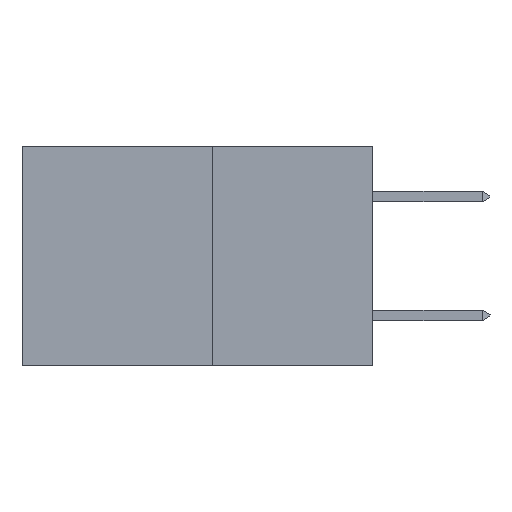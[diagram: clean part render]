
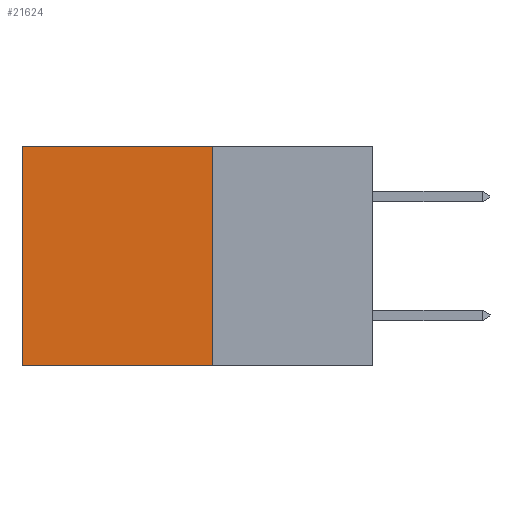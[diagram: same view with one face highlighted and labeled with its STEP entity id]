
A CAD part, left-side view. The second image highlights one B-rep face of the part: STEP entity #21624.
In plain terms, the highlighted planar face has unit normal (-1, 0, 0).
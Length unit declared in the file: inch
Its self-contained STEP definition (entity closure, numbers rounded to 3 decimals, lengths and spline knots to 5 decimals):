
#199 = CARTESIAN_POINT ( 'NONE',  ( 0.277, 0.27, 0. ) ) ;
#766 = EDGE_CURVE ( 'NONE', #6786, #12776, #12667, .T. ) ;
#1552 = DIRECTION ( 'NONE',  ( 0., 1., 0. ) ) ;
#2279 = VECTOR ( 'NONE', #3803, 39.37008 ) ;
#3022 = CARTESIAN_POINT ( 'NONE',  ( 0.277, 0.27, -0.37 ) ) ;
#3259 = CARTESIAN_POINT ( 'NONE',  ( 0.277, 0.27, 0. ) ) ;
#3731 = VECTOR ( 'NONE', #17454, 39.37008 ) ;
#3803 = DIRECTION ( 'NONE',  ( 0., 1., 0. ) ) ;
#4736 = PLANE ( 'NONE',  #23978 ) ;
#4869 = CARTESIAN_POINT ( 'NONE',  ( 0.277, 0.59, -0.37 ) ) ;
#4876 = CARTESIAN_POINT ( 'NONE',  ( 0.277, 0.27, -0.37 ) ) ;
#5575 = ORIENTED_EDGE ( 'NONE', *, *, #766, .T. ) ;
#6635 = DIRECTION ( 'NONE',  ( 0., 0., -1. ) ) ;
#6786 = VERTEX_POINT ( 'NONE', #3259 ) ;
#6839 = EDGE_CURVE ( 'NONE', #16352, #12604, #13921, .T. ) ;
#8417 = EDGE_CURVE ( 'NONE', #12776, #12604, #18519, .T. ) ;
#9029 = VECTOR ( 'NONE', #1552, 39.37008 ) ;
#10575 = EDGE_LOOP ( 'NONE', ( #21161, #20152, #13379, #5575 ) ) ;
#11410 = FACE_OUTER_BOUND ( 'NONE', #10575, .T. ) ;
#12289 = DIRECTION ( 'NONE',  ( 0., 0., -1. ) ) ;
#12604 = VERTEX_POINT ( 'NONE', #4869 ) ;
#12667 = LINE ( 'NONE', #199, #2279 ) ;
#12776 = VERTEX_POINT ( 'NONE', #18414 ) ;
#13379 = ORIENTED_EDGE ( 'NONE', *, *, #14635, .F. ) ;
#13921 = LINE ( 'NONE', #14507, #9029 ) ;
#13970 = CARTESIAN_POINT ( 'NONE',  ( 0.277, 0.27, -0.37 ) ) ;
#14507 = CARTESIAN_POINT ( 'NONE',  ( 0.277, 0.27, -0.37 ) ) ;
#14635 = EDGE_CURVE ( 'NONE', #6786, #16352, #15645, .T. ) ;
#15645 = LINE ( 'NONE', #4876, #20046 ) ;
#16352 = VERTEX_POINT ( 'NONE', #3022 ) ;
#17454 = DIRECTION ( 'NONE',  ( 0., 0., -1. ) ) ;
#17737 = DIRECTION ( 'NONE',  ( 1., 0., 0. ) ) ;
#18414 = CARTESIAN_POINT ( 'NONE',  ( 0.277, 0.59, 0. ) ) ;
#18519 = LINE ( 'NONE', #19319, #3731 ) ;
#19319 = CARTESIAN_POINT ( 'NONE',  ( 0.277, 0.59, -0.37 ) ) ;
#20046 = VECTOR ( 'NONE', #12289, 39.37008 ) ;
#20152 = ORIENTED_EDGE ( 'NONE', *, *, #6839, .F. ) ;
#21161 = ORIENTED_EDGE ( 'NONE', *, *, #8417, .T. ) ;
#21624 = ADVANCED_FACE ( 'NONE', ( #11410 ), #4736, .F. ) ;
#23978 = AXIS2_PLACEMENT_3D ( 'NONE', #13970, #17737, #6635 ) ;
